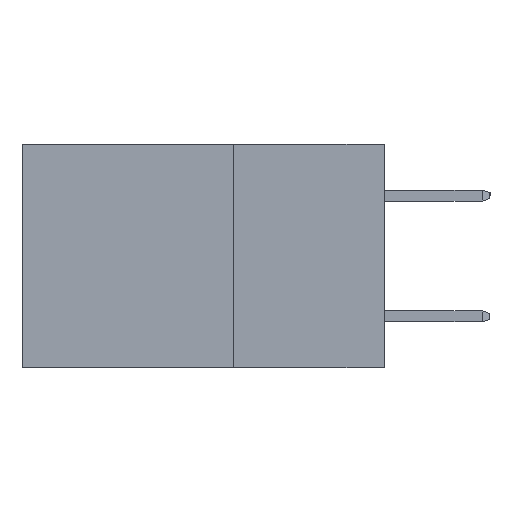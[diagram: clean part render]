
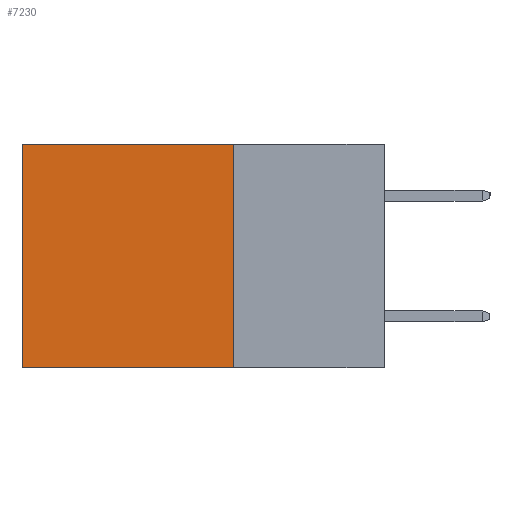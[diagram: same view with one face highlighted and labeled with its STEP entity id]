
A CAD part, left-side view. The second image highlights one B-rep face of the part: STEP entity #7230.
In plain terms, the highlighted planar face has unit normal (-1, 0, 0).
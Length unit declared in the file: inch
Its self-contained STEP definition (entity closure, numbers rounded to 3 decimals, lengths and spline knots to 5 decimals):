
#357 = VECTOR ( 'NONE', #8016, 39.37008 ) ;
#436 = CARTESIAN_POINT ( 'NONE',  ( 0.2615, 0.6, -0.37 ) ) ;
#636 = ORIENTED_EDGE ( 'NONE', *, *, #12673, .F. ) ;
#1063 = ORIENTED_EDGE ( 'NONE', *, *, #6259, .T. ) ;
#1285 = VERTEX_POINT ( 'NONE', #2301 ) ;
#1354 = DIRECTION ( 'NONE',  ( 0., 1., 0. ) ) ;
#1528 = VECTOR ( 'NONE', #14460, 39.37008 ) ;
#2301 = CARTESIAN_POINT ( 'NONE',  ( 0.2615, 0.6, -0.37 ) ) ;
#2489 = ORIENTED_EDGE ( 'NONE', *, *, #7232, .F. ) ;
#3204 = FACE_OUTER_BOUND ( 'NONE', #7046, .T. ) ;
#4397 = CARTESIAN_POINT ( 'NONE',  ( 0.2615, 0.6, 0. ) ) ;
#4673 = EDGE_CURVE ( 'NONE', #11900, #13654, #11410, .T. ) ;
#5090 = LINE ( 'NONE', #6251, #8467 ) ;
#6251 = CARTESIAN_POINT ( 'NONE',  ( 0.2615, 0.25, -0.37 ) ) ;
#6259 = EDGE_CURVE ( 'NONE', #13654, #1285, #7677, .T. ) ;
#6398 = AXIS2_PLACEMENT_3D ( 'NONE', #9140, #13967, #13875 ) ;
#6641 = PLANE ( 'NONE',  #6398 ) ;
#6806 = CARTESIAN_POINT ( 'NONE',  ( 0.2615, 0.25, 0. ) ) ;
#7046 = EDGE_LOOP ( 'NONE', ( #1063, #636, #2489, #14834 ) ) ;
#7230 = ADVANCED_FACE ( 'NONE', ( #3204 ), #6641, .F. ) ;
#7232 = EDGE_CURVE ( 'NONE', #11900, #7665, #14897, .T. ) ;
#7665 = VERTEX_POINT ( 'NONE', #8213 ) ;
#7677 = LINE ( 'NONE', #436, #1528 ) ;
#8016 = DIRECTION ( 'NONE',  ( 0., 1., 0. ) ) ;
#8213 = CARTESIAN_POINT ( 'NONE',  ( 0.2615, 0.25, -0.37 ) ) ;
#8467 = VECTOR ( 'NONE', #1354, 39.37008 ) ;
#9140 = CARTESIAN_POINT ( 'NONE',  ( 0.2615, 0.25, -0.37 ) ) ;
#11354 = DIRECTION ( 'NONE',  ( 0., 0., -1. ) ) ;
#11410 = LINE ( 'NONE', #14955, #357 ) ;
#11900 = VERTEX_POINT ( 'NONE', #6806 ) ;
#12673 = EDGE_CURVE ( 'NONE', #7665, #1285, #5090, .T. ) ;
#13266 = VECTOR ( 'NONE', #11354, 39.37008 ) ;
#13654 = VERTEX_POINT ( 'NONE', #4397 ) ;
#13875 = DIRECTION ( 'NONE',  ( 0., 0., -1. ) ) ;
#13967 = DIRECTION ( 'NONE',  ( 1., 0., 0. ) ) ;
#14460 = DIRECTION ( 'NONE',  ( 0., 0., -1. ) ) ;
#14818 = CARTESIAN_POINT ( 'NONE',  ( 0.2615, 0.25, -0.37 ) ) ;
#14834 = ORIENTED_EDGE ( 'NONE', *, *, #4673, .T. ) ;
#14897 = LINE ( 'NONE', #14818, #13266 ) ;
#14955 = CARTESIAN_POINT ( 'NONE',  ( 0.2615, 0.25, 0. ) ) ;
